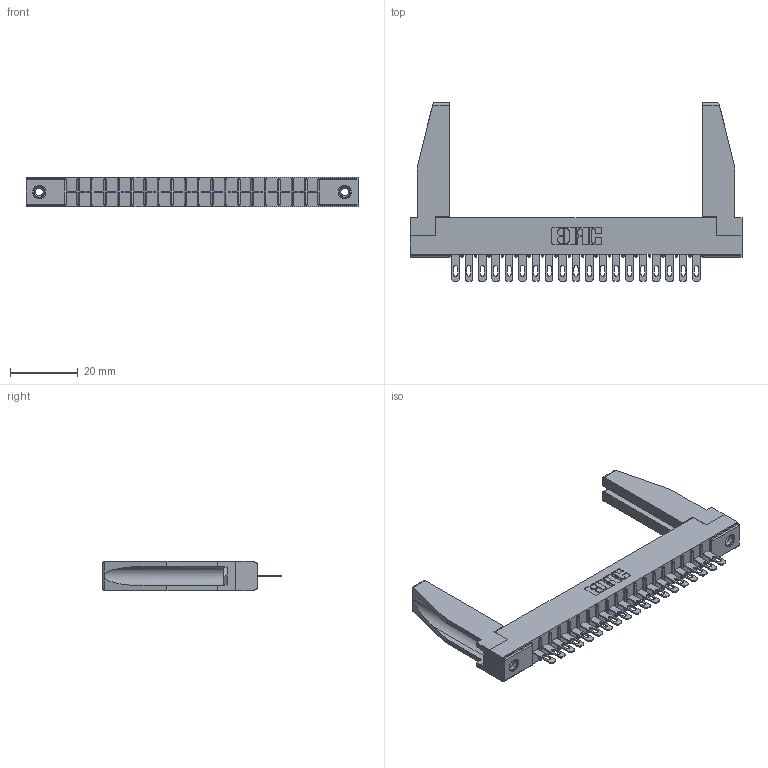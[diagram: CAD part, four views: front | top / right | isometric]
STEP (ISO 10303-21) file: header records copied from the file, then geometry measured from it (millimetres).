
FILE_DESCRIPTION (( 'STEP AP203' ), '1' );
FILE_NAME ('306-019-500-178.STEP', '2019-09-11T20:30:28', ( '' ), ( '' ), 'SwSTEP 2.0', 'SolidWorks 2016', '' );
FILE_SCHEMA (( 'CONFIG_CONTROL_DESIGN' ));
Length unit declared in the file: inch
Products named in the file (5): 306 Part_.156 Dia; 307-220-078; 345-250-001_345-250-001-102; 306-290-001_100; 306-019-500-178
Assembly tree (24 placements, depth 2):
  306-019-500-178
    306 Part_.156 Dia
    306-290-001_100  x19
    345-250-001_345-250-001-102  x2
    307-220-078  x2
Bounding box: 98.3 x 52.91 x 8.71 mm (x, y, z)
Volume: 10760 mm3; surface area: 14050.8 mm2
Topology: 24 solids, 24 shells, 1690 faces, 4731 edges, 3042 vertices
Faces by surface type: plane 1102, cylinder 496, sphere 76, cone 12, torus 4
Entity records: 23301 total; most frequent: CARTESIAN_POINT 3910, ORIENTED_EDGE 3832, DIRECTION 3810, EDGE_CURVE 1916, LINE 1486, VECTOR 1486, VERTEX_POINT 1220, AXIS2_PLACEMENT_3D 1162
